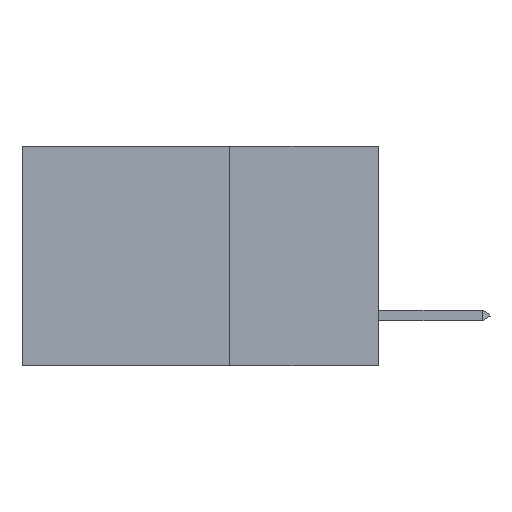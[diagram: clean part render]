
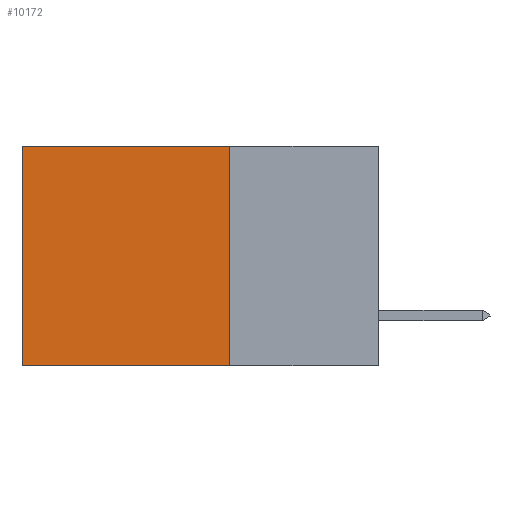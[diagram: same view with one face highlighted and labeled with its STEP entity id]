
A CAD part, left-side view. The second image highlights one B-rep face of the part: STEP entity #10172.
In plain terms, the highlighted planar face has unit normal (-1, 0, 0).
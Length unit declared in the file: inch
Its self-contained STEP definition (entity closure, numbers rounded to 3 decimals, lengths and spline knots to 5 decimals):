
#113 = CARTESIAN_POINT ( 'NONE',  ( 0.298, 0.25, 0. ) ) ;
#160 = VECTOR ( 'NONE', #12076, 39.37008 ) ;
#229 = CARTESIAN_POINT ( 'NONE',  ( 0.298, 0.25, 0. ) ) ;
#975 = ORIENTED_EDGE ( 'NONE', *, *, #7113, .T. ) ;
#1008 = EDGE_CURVE ( 'NONE', #10603, #11547, #3994, .T. ) ;
#1227 = ORIENTED_EDGE ( 'NONE', *, *, #7108, .F. ) ;
#1929 = DIRECTION ( 'NONE',  ( 0., 1., 0. ) ) ;
#2425 = DIRECTION ( 'NONE',  ( 1., 0., 0. ) ) ;
#3994 = LINE ( 'NONE', #12459, #12926 ) ;
#4767 = PLANE ( 'NONE',  #10915 ) ;
#4995 = DIRECTION ( 'NONE',  ( 0., 0., -1. ) ) ;
#5479 = ORIENTED_EDGE ( 'NONE', *, *, #10105, .T. ) ;
#6393 = VERTEX_POINT ( 'NONE', #9191 ) ;
#7083 = VECTOR ( 'NONE', #8414, 39.37008 ) ;
#7108 = EDGE_CURVE ( 'NONE', #7109, #10603, #12780, .T. ) ;
#7109 = VERTEX_POINT ( 'NONE', #229 ) ;
#7113 = EDGE_CURVE ( 'NONE', #7109, #6393, #11695, .T. ) ;
#7263 = CARTESIAN_POINT ( 'NONE',  ( 0.298, 0.25, 0. ) ) ;
#7371 = CARTESIAN_POINT ( 'NONE',  ( 0.298, 0.25, 0. ) ) ;
#7625 = CARTESIAN_POINT ( 'NONE',  ( 0.298, 0.6, -0.37 ) ) ;
#8414 = DIRECTION ( 'NONE',  ( 0., 0., -1. ) ) ;
#8957 = VECTOR ( 'NONE', #4995, 39.37008 ) ;
#9191 = CARTESIAN_POINT ( 'NONE',  ( 0.298, 0.6, 0. ) ) ;
#9356 = LINE ( 'NONE', #12018, #7083 ) ;
#9417 = CARTESIAN_POINT ( 'NONE',  ( 0.298, 0.25, -0.37 ) ) ;
#10105 = EDGE_CURVE ( 'NONE', #6393, #11547, #9356, .T. ) ;
#10172 = ADVANCED_FACE ( 'NONE', ( #11534 ), #4767, .F. ) ;
#10472 = EDGE_LOOP ( 'NONE', ( #5479, #14266, #1227, #975 ) ) ;
#10603 = VERTEX_POINT ( 'NONE', #9417 ) ;
#10915 = AXIS2_PLACEMENT_3D ( 'NONE', #113, #2425, #12967 ) ;
#11534 = FACE_OUTER_BOUND ( 'NONE', #10472, .T. ) ;
#11547 = VERTEX_POINT ( 'NONE', #7625 ) ;
#11695 = LINE ( 'NONE', #7263, #160 ) ;
#12018 = CARTESIAN_POINT ( 'NONE',  ( 0.298, 0.6, 0. ) ) ;
#12076 = DIRECTION ( 'NONE',  ( 0., 1., 0. ) ) ;
#12459 = CARTESIAN_POINT ( 'NONE',  ( 0.298, 0.25, -0.37 ) ) ;
#12780 = LINE ( 'NONE', #7371, #8957 ) ;
#12926 = VECTOR ( 'NONE', #1929, 39.37008 ) ;
#12967 = DIRECTION ( 'NONE',  ( 0., 0., -1. ) ) ;
#14266 = ORIENTED_EDGE ( 'NONE', *, *, #1008, .F. ) ;
